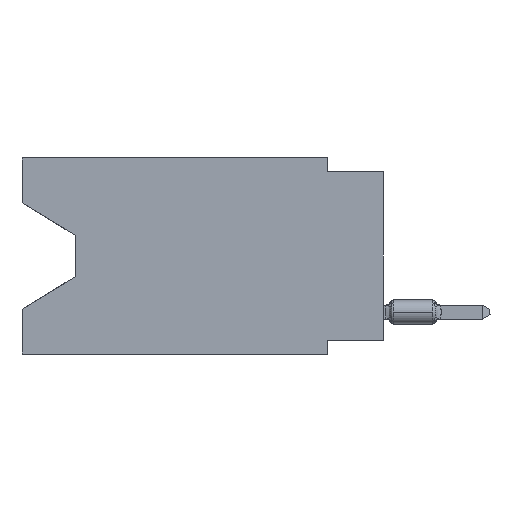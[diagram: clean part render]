
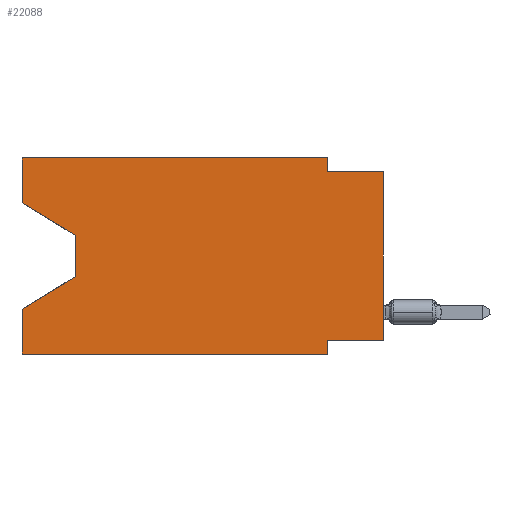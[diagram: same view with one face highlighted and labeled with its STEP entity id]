
A CAD part, left-side view. The second image highlights one B-rep face of the part: STEP entity #22088.
In plain terms, the highlighted planar face has unit normal (-1, 0, 0).
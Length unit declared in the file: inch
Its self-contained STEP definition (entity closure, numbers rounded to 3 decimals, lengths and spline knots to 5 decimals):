
#953 = VECTOR ( 'NONE', #61598, 39.37008 ) ;
#1878 = CARTESIAN_POINT ( 'NONE',  ( 0., 0.55, -0.212 ) ) ;
#2031 = EDGE_CURVE ( 'NONE', #49181, #8891, #35962, .T. ) ;
#2602 = CARTESIAN_POINT ( 'NONE',  ( 0., 0., -0.325 ) ) ;
#2643 = ORIENTED_EDGE ( 'NONE', *, *, #68991, .F. ) ;
#2720 = CARTESIAN_POINT ( 'NONE',  ( 0., 0.645, -0.35 ) ) ;
#2763 = LINE ( 'NONE', #37062, #36047 ) ;
#3428 = VERTEX_POINT ( 'NONE', #47408 ) ;
#3717 = LINE ( 'NONE', #19482, #59073 ) ;
#6161 = ORIENTED_EDGE ( 'NONE', *, *, #68178, .F. ) ;
#6703 = CARTESIAN_POINT ( 'NONE',  ( 0., 0., 0. ) ) ;
#6745 = VERTEX_POINT ( 'NONE', #2602 ) ;
#7484 = ORIENTED_EDGE ( 'NONE', *, *, #62992, .T. ) ;
#7615 = DIRECTION ( 'NONE',  ( 0., -1., 0. ) ) ;
#8891 = VERTEX_POINT ( 'NONE', #53600 ) ;
#9021 = CARTESIAN_POINT ( 'NONE',  ( 0., 0.1, 0. ) ) ;
#9172 = VECTOR ( 'NONE', #12568, 39.37008 ) ;
#9590 = ORIENTED_EDGE ( 'NONE', *, *, #15454, .F. ) ;
#10165 = CARTESIAN_POINT ( 'NONE',  ( 0., 0.645, -0.08025 ) ) ;
#10177 = CARTESIAN_POINT ( 'NONE',  ( 0., 0.55, -0.212 ) ) ;
#10812 = ORIENTED_EDGE ( 'NONE', *, *, #28163, .F. ) ;
#11457 = CARTESIAN_POINT ( 'NONE',  ( 0., 0.645, -0.35 ) ) ;
#11519 = VERTEX_POINT ( 'NONE', #10177 ) ;
#11942 = AXIS2_PLACEMENT_3D ( 'NONE', #38464, #37740, #59916 ) ;
#12568 = DIRECTION ( 'NONE',  ( 0., 0., -1. ) ) ;
#14173 = VERTEX_POINT ( 'NONE', #66559 ) ;
#14204 = CARTESIAN_POINT ( 'NONE',  ( 0., 0.645, 0. ) ) ;
#15454 = EDGE_CURVE ( 'NONE', #67053, #39927, #2763, .T. ) ;
#16154 = CARTESIAN_POINT ( 'NONE',  ( 0., 0., -0.025 ) ) ;
#16667 = PLANE ( 'NONE',  #11942 ) ;
#17549 = EDGE_CURVE ( 'NONE', #6745, #14173, #18604, .T. ) ;
#17937 = EDGE_CURVE ( 'NONE', #64999, #67053, #23193, .T. ) ;
#18336 = CARTESIAN_POINT ( 'NONE',  ( 0., 0.1, 0. ) ) ;
#18604 = LINE ( 'NONE', #40404, #68000 ) ;
#19482 = CARTESIAN_POINT ( 'NONE',  ( 0., 0.55, -0.138 ) ) ;
#20848 = VECTOR ( 'NONE', #28525, 39.37008 ) ;
#22088 = ADVANCED_FACE ( 'NONE', ( #70291 ), #16667, .F. ) ;
#22502 = DIRECTION ( 'NONE',  ( 0., 0., 1. ) ) ;
#22654 = ORIENTED_EDGE ( 'NONE', *, *, #17549, .F. ) ;
#22865 = LINE ( 'NONE', #28574, #45107 ) ;
#23193 = LINE ( 'NONE', #33923, #37196 ) ;
#24996 = ORIENTED_EDGE ( 'NONE', *, *, #2031, .T. ) ;
#25637 = DIRECTION ( 'NONE',  ( 0., 0., 1. ) ) ;
#26147 = VERTEX_POINT ( 'NONE', #54931 ) ;
#28163 = EDGE_CURVE ( 'NONE', #3428, #55052, #56595, .T. ) ;
#28525 = DIRECTION ( 'NONE',  ( 0., 0., 1. ) ) ;
#28574 = CARTESIAN_POINT ( 'NONE',  ( 0., 0.645, -0.08025 ) ) ;
#29570 = DIRECTION ( 'NONE',  ( 0., -1., 0. ) ) ;
#31674 = EDGE_CURVE ( 'NONE', #69968, #11519, #3717, .T. ) ;
#33923 = CARTESIAN_POINT ( 'NONE',  ( 0., 0.645, 0. ) ) ;
#34107 = CARTESIAN_POINT ( 'NONE',  ( 0., 0.55, -0.138 ) ) ;
#35962 = LINE ( 'NONE', #2720, #47679 ) ;
#36047 = VECTOR ( 'NONE', #63898, 39.37008 ) ;
#36349 = CARTESIAN_POINT ( 'NONE',  ( 0., 0.645, 0. ) ) ;
#37062 = CARTESIAN_POINT ( 'NONE',  ( 0., 0.645, 0. ) ) ;
#37196 = VECTOR ( 'NONE', #22502, 39.37008 ) ;
#37740 = DIRECTION ( 'NONE',  ( 1., 0., 0. ) ) ;
#38464 = CARTESIAN_POINT ( 'NONE',  ( 0., 0.645, 0. ) ) ;
#39056 = ORIENTED_EDGE ( 'NONE', *, *, #17937, .F. ) ;
#39927 = VERTEX_POINT ( 'NONE', #18336 ) ;
#40146 = CARTESIAN_POINT ( 'NONE',  ( 0., 0., -0.025 ) ) ;
#40404 = CARTESIAN_POINT ( 'NONE',  ( 0., 0., -0.325 ) ) ;
#45107 = VECTOR ( 'NONE', #60040, 39.37008 ) ;
#46531 = ORIENTED_EDGE ( 'NONE', *, *, #31674, .T. ) ;
#47090 = LINE ( 'NONE', #36349, #50429 ) ;
#47408 = CARTESIAN_POINT ( 'NONE',  ( 0., 0.1, -0.025 ) ) ;
#47679 = VECTOR ( 'NONE', #29570, 39.37008 ) ;
#49181 = VERTEX_POINT ( 'NONE', #11457 ) ;
#49642 = ORIENTED_EDGE ( 'NONE', *, *, #65488, .F. ) ;
#49764 = EDGE_CURVE ( 'NONE', #6745, #55052, #55692, .T. ) ;
#49765 = LINE ( 'NONE', #66919, #9172 ) ;
#50111 = VECTOR ( 'NONE', #7615, 39.37008 ) ;
#50429 = VECTOR ( 'NONE', #25637, 39.37008 ) ;
#51233 = LINE ( 'NONE', #1878, #953 ) ;
#52288 = LINE ( 'NONE', #9021, #69828 ) ;
#52632 = DIRECTION ( 'NONE',  ( 0., 0., -1. ) ) ;
#53600 = CARTESIAN_POINT ( 'NONE',  ( 0., 0.1, -0.35 ) ) ;
#54322 = EDGE_CURVE ( 'NONE', #64999, #69968, #22865, .T. ) ;
#54931 = CARTESIAN_POINT ( 'NONE',  ( 0., 0.645, -0.26975 ) ) ;
#55052 = VERTEX_POINT ( 'NONE', #16154 ) ;
#55095 = DIRECTION ( 'NONE',  ( 0., 1., 0. ) ) ;
#55692 = LINE ( 'NONE', #6703, #20848 ) ;
#56486 = ORIENTED_EDGE ( 'NONE', *, *, #54322, .T. ) ;
#56595 = LINE ( 'NONE', #40146, #50111 ) ;
#59073 = VECTOR ( 'NONE', #63088, 39.37008 ) ;
#59355 = EDGE_LOOP ( 'NONE', ( #56486, #46531, #7484, #6161, #24996, #49642, #22654, #68205, #10812, #2643, #9590, #39056 ) ) ;
#59916 = DIRECTION ( 'NONE',  ( 0., 0., -1. ) ) ;
#60040 = DIRECTION ( 'NONE',  ( 0., -0.855, -0.519 ) ) ;
#61598 = DIRECTION ( 'NONE',  ( 0., 0.855, -0.519 ) ) ;
#62992 = EDGE_CURVE ( 'NONE', #11519, #26147, #51233, .T. ) ;
#63088 = DIRECTION ( 'NONE',  ( 0., 0., -1. ) ) ;
#63898 = DIRECTION ( 'NONE',  ( 0., -1., 0. ) ) ;
#64999 = VERTEX_POINT ( 'NONE', #10165 ) ;
#65488 = EDGE_CURVE ( 'NONE', #14173, #8891, #49765, .T. ) ;
#66559 = CARTESIAN_POINT ( 'NONE',  ( 0., 0.1, -0.325 ) ) ;
#66919 = CARTESIAN_POINT ( 'NONE',  ( 0., 0.1, -0.35 ) ) ;
#67053 = VERTEX_POINT ( 'NONE', #14204 ) ;
#68000 = VECTOR ( 'NONE', #55095, 39.37008 ) ;
#68178 = EDGE_CURVE ( 'NONE', #49181, #26147, #47090, .T. ) ;
#68205 = ORIENTED_EDGE ( 'NONE', *, *, #49764, .T. ) ;
#68991 = EDGE_CURVE ( 'NONE', #39927, #3428, #52288, .T. ) ;
#69828 = VECTOR ( 'NONE', #52632, 39.37008 ) ;
#69968 = VERTEX_POINT ( 'NONE', #34107 ) ;
#70291 = FACE_OUTER_BOUND ( 'NONE', #59355, .T. ) ;
